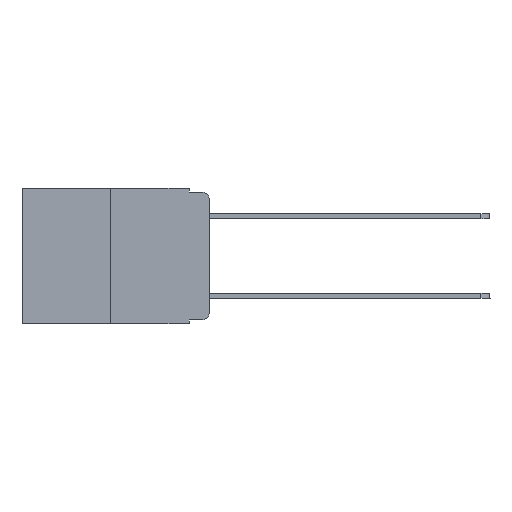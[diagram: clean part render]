
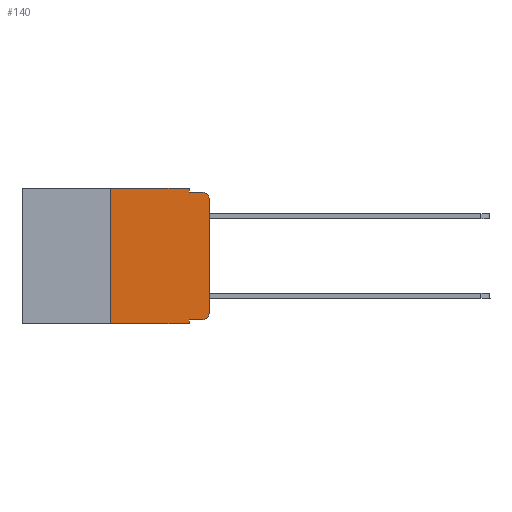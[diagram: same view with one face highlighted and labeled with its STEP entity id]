
A CAD part, left-side view. The second image highlights one B-rep face of the part: STEP entity #140.
In plain terms, the highlighted planar face has unit normal (-1, 0, 0).
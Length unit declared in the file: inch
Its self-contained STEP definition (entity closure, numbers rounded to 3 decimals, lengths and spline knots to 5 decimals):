
#65 = DIRECTION ( 'NONE',  ( 0., 0., 1. ) ) ;
#93 = DIRECTION ( 'NONE',  ( 0., 0., -1. ) ) ;
#140 = ADVANCED_FACE ( 'NONE', ( #4623 ), #5013, .F. ) ;
#310 = VECTOR ( 'NONE', #2152, 39.37008 ) ;
#335 = EDGE_CURVE ( 'NONE', #14565, #3092, #9169, .T. ) ;
#441 = ORIENTED_EDGE ( 'NONE', *, *, #8560, .T. ) ;
#625 = CARTESIAN_POINT ( 'NONE',  ( 0., 0.473, 0. ) ) ;
#825 = CIRCLE ( 'NONE', #2719, 0.02 ) ;
#1086 = VECTOR ( 'NONE', #65, 39.37008 ) ;
#1458 = VECTOR ( 'NONE', #93, 39.37008 ) ;
#2115 = CARTESIAN_POINT ( 'NONE',  ( 0., 0.051, -0.333 ) ) ;
#2152 = DIRECTION ( 'NONE',  ( 0., -1., 0. ) ) ;
#2396 = DIRECTION ( 'NONE',  ( 0., -1., 0. ) ) ;
#2473 = EDGE_CURVE ( 'NONE', #7034, #9645, #825, .T. ) ;
#2526 = EDGE_CURVE ( 'NONE', #13192, #13435, #15576, .T. ) ;
#2552 = CARTESIAN_POINT ( 'NONE',  ( 0., 0., 0. ) ) ;
#2688 = DIRECTION ( 'NONE',  ( 0., 0., -1. ) ) ;
#2719 = AXIS2_PLACEMENT_3D ( 'NONE', #4755, #8743, #7283 ) ;
#3029 = LINE ( 'NONE', #3671, #1458 ) ;
#3092 = VERTEX_POINT ( 'NONE', #7952 ) ;
#3199 = CARTESIAN_POINT ( 'NONE',  ( 0., 0.25, 0. ) ) ;
#3335 = EDGE_LOOP ( 'NONE', ( #441, #12616, #8493, #8595, #10585, #9810, #11916, #12301, #7673, #5295 ) ) ;
#3431 = EDGE_CURVE ( 'NONE', #7101, #13861, #5623, .T. ) ;
#3614 = VERTEX_POINT ( 'NONE', #14157 ) ;
#3625 = DIRECTION ( 'NONE',  ( 1., 0., 0. ) ) ;
#3652 = LINE ( 'NONE', #9708, #310 ) ;
#3671 = CARTESIAN_POINT ( 'NONE',  ( 0., 0.051, 0. ) ) ;
#3681 = CARTESIAN_POINT ( 'NONE',  ( 0., 0.02, -0.313 ) ) ;
#4549 = VERTEX_POINT ( 'NONE', #6877 ) ;
#4594 = DIRECTION ( 'NONE',  ( 0., -1., 0. ) ) ;
#4623 = FACE_OUTER_BOUND ( 'NONE', #3335, .T. ) ;
#4755 = CARTESIAN_POINT ( 'NONE',  ( 0., 0.02, -0.03 ) ) ;
#4954 = VECTOR ( 'NONE', #7587, 39.37008 ) ;
#5013 = PLANE ( 'NONE',  #13770 ) ;
#5143 = CARTESIAN_POINT ( 'NONE',  ( 0., 0., -0.03 ) ) ;
#5229 = EDGE_CURVE ( 'NONE', #13435, #3614, #3029, .T. ) ;
#5295 = ORIENTED_EDGE ( 'NONE', *, *, #335, .T. ) ;
#5623 = LINE ( 'NONE', #7196, #6815 ) ;
#5651 = DIRECTION ( 'NONE',  ( 0., 0., 1. ) ) ;
#6111 = VECTOR ( 'NONE', #2396, 39.37008 ) ;
#6367 = VECTOR ( 'NONE', #4594, 39.37008 ) ;
#6815 = VECTOR ( 'NONE', #8426, 39.37008 ) ;
#6877 = CARTESIAN_POINT ( 'NONE',  ( 0., 0.25, -0.343 ) ) ;
#7034 = VERTEX_POINT ( 'NONE', #5143 ) ;
#7101 = VERTEX_POINT ( 'NONE', #11789 ) ;
#7196 = CARTESIAN_POINT ( 'NONE',  ( 0., 0.051, 0. ) ) ;
#7206 = AXIS2_PLACEMENT_3D ( 'NONE', #3681, #12695, #8662 ) ;
#7283 = DIRECTION ( 'NONE',  ( 0., 0., -1. ) ) ;
#7587 = DIRECTION ( 'NONE',  ( 0., -1., 0. ) ) ;
#7673 = ORIENTED_EDGE ( 'NONE', *, *, #11225, .T. ) ;
#7738 = CARTESIAN_POINT ( 'NONE',  ( 0., 0.051, 0. ) ) ;
#7802 = EDGE_CURVE ( 'NONE', #4549, #13192, #12162, .T. ) ;
#7952 = CARTESIAN_POINT ( 'NONE',  ( 0., 0., -0.313 ) ) ;
#8327 = LINE ( 'NONE', #8800, #4954 ) ;
#8426 = DIRECTION ( 'NONE',  ( 0., 0., -1. ) ) ;
#8493 = ORIENTED_EDGE ( 'NONE', *, *, #12767, .F. ) ;
#8560 = EDGE_CURVE ( 'NONE', #3092, #7034, #12342, .T. ) ;
#8595 = ORIENTED_EDGE ( 'NONE', *, *, #5229, .F. ) ;
#8662 = DIRECTION ( 'NONE',  ( 0., 0., -1. ) ) ;
#8723 = CARTESIAN_POINT ( 'NONE',  ( 0., 0.051, -0.343 ) ) ;
#8743 = DIRECTION ( 'NONE',  ( -1., 0., 0. ) ) ;
#8800 = CARTESIAN_POINT ( 'NONE',  ( 0., 0.051, -0.01 ) ) ;
#9169 = CIRCLE ( 'NONE', #7206, 0.02 ) ;
#9645 = VERTEX_POINT ( 'NONE', #14978 ) ;
#9708 = CARTESIAN_POINT ( 'NONE',  ( 0., 0.473, -0.343 ) ) ;
#9810 = ORIENTED_EDGE ( 'NONE', *, *, #7802, .F. ) ;
#10585 = ORIENTED_EDGE ( 'NONE', *, *, #2526, .F. ) ;
#10794 = EDGE_CURVE ( 'NONE', #4549, #13861, #3652, .T. ) ;
#11225 = EDGE_CURVE ( 'NONE', #7101, #14565, #14289, .T. ) ;
#11789 = CARTESIAN_POINT ( 'NONE',  ( 0., 0.051, -0.333 ) ) ;
#11916 = ORIENTED_EDGE ( 'NONE', *, *, #10794, .T. ) ;
#12162 = LINE ( 'NONE', #3199, #13513 ) ;
#12301 = ORIENTED_EDGE ( 'NONE', *, *, #3431, .F. ) ;
#12342 = LINE ( 'NONE', #2552, #1086 ) ;
#12616 = ORIENTED_EDGE ( 'NONE', *, *, #2473, .T. ) ;
#12695 = DIRECTION ( 'NONE',  ( -1., 0., 0. ) ) ;
#12767 = EDGE_CURVE ( 'NONE', #3614, #9645, #8327, .T. ) ;
#13192 = VERTEX_POINT ( 'NONE', #14522 ) ;
#13435 = VERTEX_POINT ( 'NONE', #7738 ) ;
#13513 = VECTOR ( 'NONE', #5651, 39.37008 ) ;
#13637 = CARTESIAN_POINT ( 'NONE',  ( 0., 0.02, -0.333 ) ) ;
#13770 = AXIS2_PLACEMENT_3D ( 'NONE', #625, #3625, #2688 ) ;
#13861 = VERTEX_POINT ( 'NONE', #8723 ) ;
#14157 = CARTESIAN_POINT ( 'NONE',  ( 0., 0.051, -0.01 ) ) ;
#14289 = LINE ( 'NONE', #2115, #6367 ) ;
#14522 = CARTESIAN_POINT ( 'NONE',  ( 0., 0.25, 0. ) ) ;
#14565 = VERTEX_POINT ( 'NONE', #13637 ) ;
#14909 = CARTESIAN_POINT ( 'NONE',  ( 0., 0.473, 0. ) ) ;
#14978 = CARTESIAN_POINT ( 'NONE',  ( 0., 0.02, -0.01 ) ) ;
#15576 = LINE ( 'NONE', #14909, #6111 ) ;
